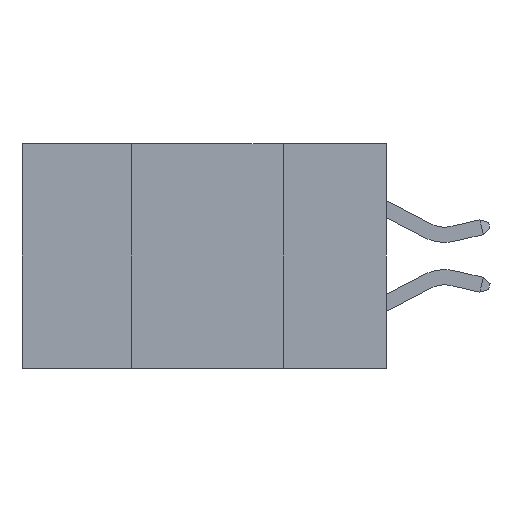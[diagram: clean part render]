
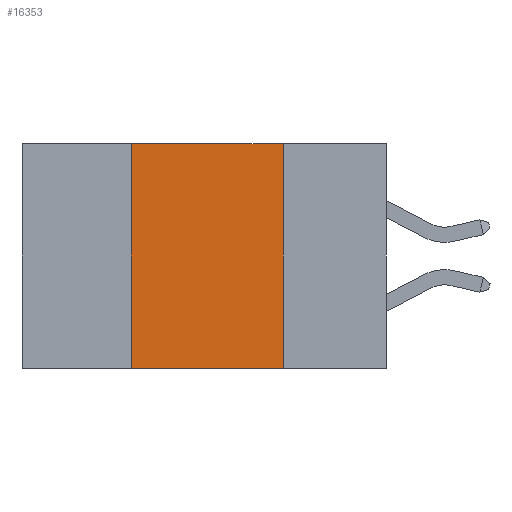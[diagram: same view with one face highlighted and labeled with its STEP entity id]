
A CAD part, left-side view. The second image highlights one B-rep face of the part: STEP entity #16353.
In plain terms, the highlighted planar face has unit normal (-1, 0, 0).
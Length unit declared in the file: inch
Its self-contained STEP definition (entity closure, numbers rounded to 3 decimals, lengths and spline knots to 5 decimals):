
#921 = AXIS2_PLACEMENT_3D ( 'NONE', #4983, #19568, #19650 ) ;
#927 = CARTESIAN_POINT ( 'NONE',  ( 0., 0.17, 0. ) ) ;
#2476 = VERTEX_POINT ( 'NONE', #7226 ) ;
#2887 = VECTOR ( 'NONE', #21623, 39.37008 ) ;
#3027 = CARTESIAN_POINT ( 'NONE',  ( 0., 0.6, 0. ) ) ;
#3656 = VERTEX_POINT ( 'NONE', #11100 ) ;
#3797 = DIRECTION ( 'NONE',  ( 0., 0., 1. ) ) ;
#4094 = EDGE_LOOP ( 'NONE', ( #18031, #14418, #9322, #15764 ) ) ;
#4430 = VECTOR ( 'NONE', #3797, 39.37008 ) ;
#4644 = CARTESIAN_POINT ( 'NONE',  ( 0., 0.6, -0.37 ) ) ;
#4718 = DIRECTION ( 'NONE',  ( 0., -1., 0. ) ) ;
#4983 = CARTESIAN_POINT ( 'NONE',  ( 0., 0.6, 0. ) ) ;
#5008 = LINE ( 'NONE', #14837, #4430 ) ;
#5294 = CARTESIAN_POINT ( 'NONE',  ( 0., 0.17, 0. ) ) ;
#7226 = CARTESIAN_POINT ( 'NONE',  ( 0., 0.17, -0.37 ) ) ;
#8306 = VERTEX_POINT ( 'NONE', #927 ) ;
#8315 = EDGE_CURVE ( 'NONE', #3656, #2476, #8955, .T. ) ;
#8391 = EDGE_CURVE ( 'NONE', #10902, #8306, #20186, .T. ) ;
#8647 = VECTOR ( 'NONE', #4718, 39.37008 ) ;
#8955 = LINE ( 'NONE', #4644, #22410 ) ;
#9322 = ORIENTED_EDGE ( 'NONE', *, *, #20130, .F. ) ;
#10902 = VERTEX_POINT ( 'NONE', #21908 ) ;
#11100 = CARTESIAN_POINT ( 'NONE',  ( 0., 0.42, -0.37 ) ) ;
#12231 = DIRECTION ( 'NONE',  ( 0., -1., 0. ) ) ;
#12983 = LINE ( 'NONE', #5294, #2887 ) ;
#14418 = ORIENTED_EDGE ( 'NONE', *, *, #8391, .F. ) ;
#14837 = CARTESIAN_POINT ( 'NONE',  ( 0., 0.42, 0. ) ) ;
#15764 = ORIENTED_EDGE ( 'NONE', *, *, #8315, .T. ) ;
#16353 = ADVANCED_FACE ( 'NONE', ( #21592 ), #19413, .F. ) ;
#16417 = EDGE_CURVE ( 'NONE', #8306, #2476, #12983, .T. ) ;
#18031 = ORIENTED_EDGE ( 'NONE', *, *, #16417, .F. ) ;
#19413 = PLANE ( 'NONE',  #921 ) ;
#19568 = DIRECTION ( 'NONE',  ( 1., 0., 0. ) ) ;
#19650 = DIRECTION ( 'NONE',  ( 0., 0., -1. ) ) ;
#20130 = EDGE_CURVE ( 'NONE', #3656, #10902, #5008, .T. ) ;
#20186 = LINE ( 'NONE', #3027, #8647 ) ;
#21592 = FACE_OUTER_BOUND ( 'NONE', #4094, .T. ) ;
#21623 = DIRECTION ( 'NONE',  ( 0., 0., -1. ) ) ;
#21908 = CARTESIAN_POINT ( 'NONE',  ( 0., 0.42, 0. ) ) ;
#22410 = VECTOR ( 'NONE', #12231, 39.37008 ) ;
